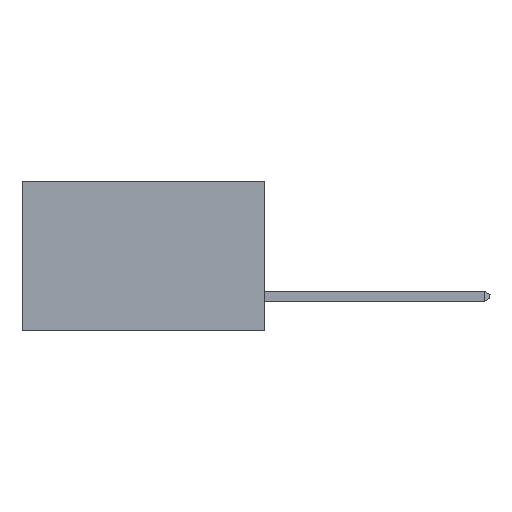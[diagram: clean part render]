
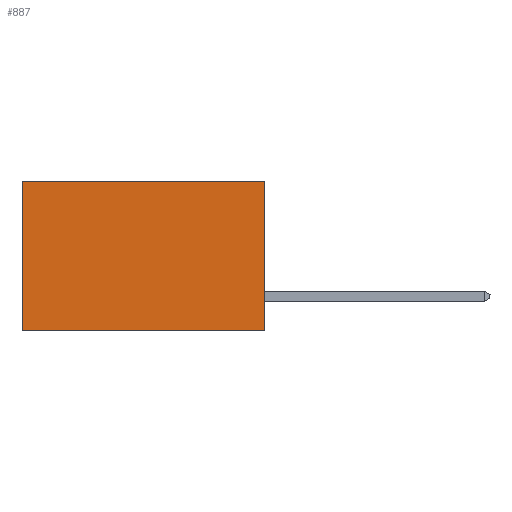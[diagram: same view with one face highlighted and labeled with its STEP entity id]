
A CAD part, left-side view. The second image highlights one B-rep face of the part: STEP entity #887.
In plain terms, the highlighted planar face has unit normal (-1, 0, 0).
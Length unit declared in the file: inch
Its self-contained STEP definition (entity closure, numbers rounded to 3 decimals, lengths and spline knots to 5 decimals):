
#887 = ADVANCED_FACE ( 'NONE', ( #5870 ), #15817, .F. ) ;
#2245 = CARTESIAN_POINT ( 'NONE',  ( 0.2615, 0., -0.37 ) ) ;
#2545 = ORIENTED_EDGE ( 'NONE', *, *, #5474, .T. ) ;
#2810 = AXIS2_PLACEMENT_3D ( 'NONE', #4504, #17115, #3222 ) ;
#2837 = ORIENTED_EDGE ( 'NONE', *, *, #15799, .F. ) ;
#3050 = CARTESIAN_POINT ( 'NONE',  ( 0.2615, 0., 0. ) ) ;
#3222 = DIRECTION ( 'NONE',  ( 0., 0., -1. ) ) ;
#4504 = CARTESIAN_POINT ( 'NONE',  ( 0.2615, 0., -0.37 ) ) ;
#4615 = VECTOR ( 'NONE', #9953, 39.37008 ) ;
#5441 = LINE ( 'NONE', #13654, #12290 ) ;
#5474 = EDGE_CURVE ( 'NONE', #13252, #6771, #9181, .T. ) ;
#5870 = FACE_OUTER_BOUND ( 'NONE', #16307, .T. ) ;
#6771 = VERTEX_POINT ( 'NONE', #17854 ) ;
#7575 = ORIENTED_EDGE ( 'NONE', *, *, #12587, .T. ) ;
#9091 = CARTESIAN_POINT ( 'NONE',  ( 0.2615, 0.6, -0.37 ) ) ;
#9181 = LINE ( 'NONE', #9091, #15811 ) ;
#9344 = DIRECTION ( 'NONE',  ( 0., 1., 0. ) ) ;
#9702 = VERTEX_POINT ( 'NONE', #14206 ) ;
#9855 = CARTESIAN_POINT ( 'NONE',  ( 0.2615, 0., 0. ) ) ;
#9953 = DIRECTION ( 'NONE',  ( 0., 1., 0. ) ) ;
#10039 = LINE ( 'NONE', #3050, #4615 ) ;
#10467 = LINE ( 'NONE', #2245, #13507 ) ;
#12114 = EDGE_CURVE ( 'NONE', #15253, #9702, #5441, .T. ) ;
#12290 = VECTOR ( 'NONE', #15311, 39.37008 ) ;
#12587 = EDGE_CURVE ( 'NONE', #15253, #13252, #10039, .T. ) ;
#13252 = VERTEX_POINT ( 'NONE', #17934 ) ;
#13507 = VECTOR ( 'NONE', #9344, 39.37008 ) ;
#13654 = CARTESIAN_POINT ( 'NONE',  ( 0.2615, 0., -0.37 ) ) ;
#14206 = CARTESIAN_POINT ( 'NONE',  ( 0.2615, 0., -0.37 ) ) ;
#14808 = ORIENTED_EDGE ( 'NONE', *, *, #12114, .F. ) ;
#15253 = VERTEX_POINT ( 'NONE', #9855 ) ;
#15311 = DIRECTION ( 'NONE',  ( 0., 0., -1. ) ) ;
#15799 = EDGE_CURVE ( 'NONE', #9702, #6771, #10467, .T. ) ;
#15811 = VECTOR ( 'NONE', #17840, 39.37008 ) ;
#15817 = PLANE ( 'NONE',  #2810 ) ;
#16307 = EDGE_LOOP ( 'NONE', ( #2545, #2837, #14808, #7575 ) ) ;
#17115 = DIRECTION ( 'NONE',  ( 1., 0., 0. ) ) ;
#17840 = DIRECTION ( 'NONE',  ( 0., 0., -1. ) ) ;
#17854 = CARTESIAN_POINT ( 'NONE',  ( 0.2615, 0.6, -0.37 ) ) ;
#17934 = CARTESIAN_POINT ( 'NONE',  ( 0.2615, 0.6, 0. ) ) ;
